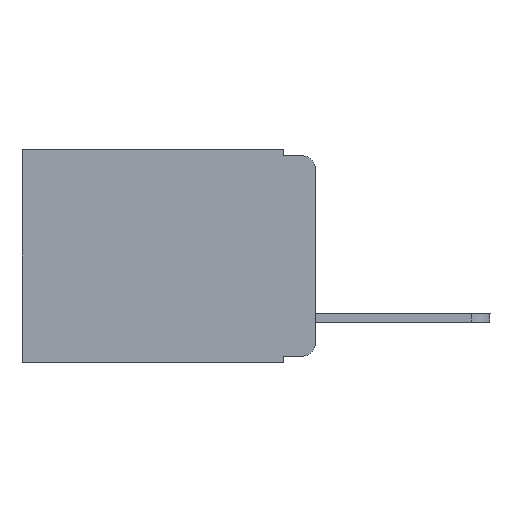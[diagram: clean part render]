
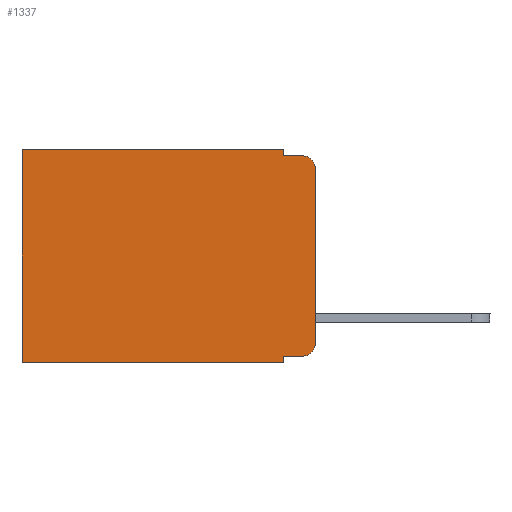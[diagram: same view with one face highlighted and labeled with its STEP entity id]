
A CAD part, left-side view. The second image highlights one B-rep face of the part: STEP entity #1337.
In plain terms, the highlighted planar face has unit normal (-1, 0, 0).
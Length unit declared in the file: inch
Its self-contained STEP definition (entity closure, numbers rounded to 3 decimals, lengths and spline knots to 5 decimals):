
#263 = LINE ( 'NONE', #3833, #11159 ) ;
#429 = CARTESIAN_POINT ( 'NONE',  ( 0.298, 0.02, -0.333 ) ) ;
#539 = DIRECTION ( 'NONE',  ( 0., 1., 0. ) ) ;
#669 = VERTEX_POINT ( 'NONE', #10972 ) ;
#685 = VERTEX_POINT ( 'NONE', #9181 ) ;
#720 = VERTEX_POINT ( 'NONE', #7597 ) ;
#746 = VERTEX_POINT ( 'NONE', #9292 ) ;
#839 = VECTOR ( 'NONE', #6575, 39.37008 ) ;
#930 = VERTEX_POINT ( 'NONE', #9744 ) ;
#1016 = AXIS2_PLACEMENT_3D ( 'NONE', #3245, #1560, #2177 ) ;
#1075 = EDGE_CURVE ( 'NONE', #10710, #9410, #263, .T. ) ;
#1337 = ADVANCED_FACE ( 'NONE', ( #3419 ), #6765, .F. ) ;
#1389 = LINE ( 'NONE', #4931, #4148 ) ;
#1391 = DIRECTION ( 'NONE',  ( 0., 0., -1. ) ) ;
#1460 = ORIENTED_EDGE ( 'NONE', *, *, #8273, .T. ) ;
#1480 = AXIS2_PLACEMENT_3D ( 'NONE', #6937, #10501, #10324 ) ;
#1560 = DIRECTION ( 'NONE',  ( -1., 0., 0. ) ) ;
#1607 = VERTEX_POINT ( 'NONE', #429 ) ;
#1686 = ORIENTED_EDGE ( 'NONE', *, *, #1075, .F. ) ;
#2013 = VECTOR ( 'NONE', #5579, 39.37008 ) ;
#2029 = CARTESIAN_POINT ( 'NONE',  ( 0.298, 0.473, 0. ) ) ;
#2119 = EDGE_CURVE ( 'NONE', #685, #1607, #6912, .T. ) ;
#2177 = DIRECTION ( 'NONE',  ( 0., 0., -1. ) ) ;
#3047 = LINE ( 'NONE', #5012, #839 ) ;
#3074 = AXIS2_PLACEMENT_3D ( 'NONE', #10326, #6819, #10199 ) ;
#3245 = CARTESIAN_POINT ( 'NONE',  ( 0.298, 0.02, -0.03 ) ) ;
#3325 = ORIENTED_EDGE ( 'NONE', *, *, #9295, .T. ) ;
#3419 = FACE_OUTER_BOUND ( 'NONE', #11231, .T. ) ;
#3690 = VECTOR ( 'NONE', #10294, 39.37008 ) ;
#3833 = CARTESIAN_POINT ( 'NONE',  ( 0.298, 0.051, 0. ) ) ;
#4148 = VECTOR ( 'NONE', #11147, 39.37008 ) ;
#4261 = LINE ( 'NONE', #9363, #8145 ) ;
#4370 = VECTOR ( 'NONE', #1391, 39.37008 ) ;
#4527 = EDGE_CURVE ( 'NONE', #9410, #10208, #4898, .T. ) ;
#4536 = EDGE_CURVE ( 'NONE', #10710, #746, #4261, .T. ) ;
#4898 = LINE ( 'NONE', #6688, #5549 ) ;
#4931 = CARTESIAN_POINT ( 'NONE',  ( 0.298, 0., -0.343 ) ) ;
#5012 = CARTESIAN_POINT ( 'NONE',  ( 0.298, 0.051, 0. ) ) ;
#5325 = VERTEX_POINT ( 'NONE', #6758 ) ;
#5549 = VECTOR ( 'NONE', #8486, 39.37008 ) ;
#5579 = DIRECTION ( 'NONE',  ( 0., 0., -1. ) ) ;
#6575 = DIRECTION ( 'NONE',  ( 0., 0., -1. ) ) ;
#6615 = ORIENTED_EDGE ( 'NONE', *, *, #2119, .T. ) ;
#6688 = CARTESIAN_POINT ( 'NONE',  ( 0.298, 0.051, -0.01 ) ) ;
#6730 = CARTESIAN_POINT ( 'NONE',  ( 0.298, 0., 0. ) ) ;
#6758 = CARTESIAN_POINT ( 'NONE',  ( 0.298, 0.473, -0.343 ) ) ;
#6765 = PLANE ( 'NONE',  #1480 ) ;
#6789 = ORIENTED_EDGE ( 'NONE', *, *, #9401, .T. ) ;
#6819 = DIRECTION ( 'NONE',  ( -1., 0., 0. ) ) ;
#6912 = LINE ( 'NONE', #9593, #3690 ) ;
#6937 = CARTESIAN_POINT ( 'NONE',  ( 0.298, 0., 0. ) ) ;
#7336 = DIRECTION ( 'NONE',  ( 0., 0., -1. ) ) ;
#7510 = ORIENTED_EDGE ( 'NONE', *, *, #8870, .F. ) ;
#7597 = CARTESIAN_POINT ( 'NONE',  ( 0.298, 0.051, -0.343 ) ) ;
#7635 = EDGE_CURVE ( 'NONE', #720, #5325, #1389, .T. ) ;
#7809 = ORIENTED_EDGE ( 'NONE', *, *, #7635, .F. ) ;
#8145 = VECTOR ( 'NONE', #539, 39.37008 ) ;
#8273 = EDGE_CURVE ( 'NONE', #746, #5325, #9783, .T. ) ;
#8409 = LINE ( 'NONE', #6730, #4370 ) ;
#8486 = DIRECTION ( 'NONE',  ( 0., -1., 0. ) ) ;
#8548 = ORIENTED_EDGE ( 'NONE', *, *, #4527, .F. ) ;
#8751 = CARTESIAN_POINT ( 'NONE',  ( 0.298, 0.051, -0.01 ) ) ;
#8870 = EDGE_CURVE ( 'NONE', #930, #669, #8409, .T. ) ;
#9181 = CARTESIAN_POINT ( 'NONE',  ( 0.298, 0.051, -0.333 ) ) ;
#9245 = CARTESIAN_POINT ( 'NONE',  ( 0.298, 0.02, -0.01 ) ) ;
#9292 = CARTESIAN_POINT ( 'NONE',  ( 0.298, 0.473, 0. ) ) ;
#9295 = EDGE_CURVE ( 'NONE', #1607, #669, #9370, .T. ) ;
#9363 = CARTESIAN_POINT ( 'NONE',  ( 0.298, 0., 0. ) ) ;
#9370 = CIRCLE ( 'NONE', #3074, 0.02 ) ;
#9401 = EDGE_CURVE ( 'NONE', #930, #10208, #10116, .T. ) ;
#9410 = VERTEX_POINT ( 'NONE', #8751 ) ;
#9593 = CARTESIAN_POINT ( 'NONE',  ( 0.298, 0.051, -0.333 ) ) ;
#9738 = EDGE_CURVE ( 'NONE', #685, #720, #3047, .T. ) ;
#9744 = CARTESIAN_POINT ( 'NONE',  ( 0.298, 0., -0.03 ) ) ;
#9783 = LINE ( 'NONE', #2029, #2013 ) ;
#10116 = CIRCLE ( 'NONE', #1016, 0.02 ) ;
#10199 = DIRECTION ( 'NONE',  ( 0., 0., -1. ) ) ;
#10208 = VERTEX_POINT ( 'NONE', #9245 ) ;
#10294 = DIRECTION ( 'NONE',  ( 0., -1., 0. ) ) ;
#10324 = DIRECTION ( 'NONE',  ( 0., 0., -1. ) ) ;
#10326 = CARTESIAN_POINT ( 'NONE',  ( 0.298, 0.02, -0.313 ) ) ;
#10501 = DIRECTION ( 'NONE',  ( 1., 0., 0. ) ) ;
#10523 = ORIENTED_EDGE ( 'NONE', *, *, #9738, .F. ) ;
#10677 = CARTESIAN_POINT ( 'NONE',  ( 0.298, 0.051, 0. ) ) ;
#10710 = VERTEX_POINT ( 'NONE', #10677 ) ;
#10972 = CARTESIAN_POINT ( 'NONE',  ( 0.298, 0., -0.313 ) ) ;
#11147 = DIRECTION ( 'NONE',  ( 0., 1., 0. ) ) ;
#11159 = VECTOR ( 'NONE', #7336, 39.37008 ) ;
#11231 = EDGE_LOOP ( 'NONE', ( #7510, #6789, #8548, #1686, #11285, #1460, #7809, #10523, #6615, #3325 ) ) ;
#11285 = ORIENTED_EDGE ( 'NONE', *, *, #4536, .T. ) ;
